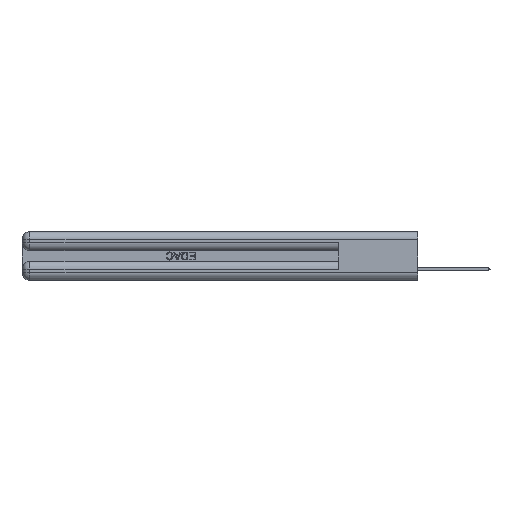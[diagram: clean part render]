
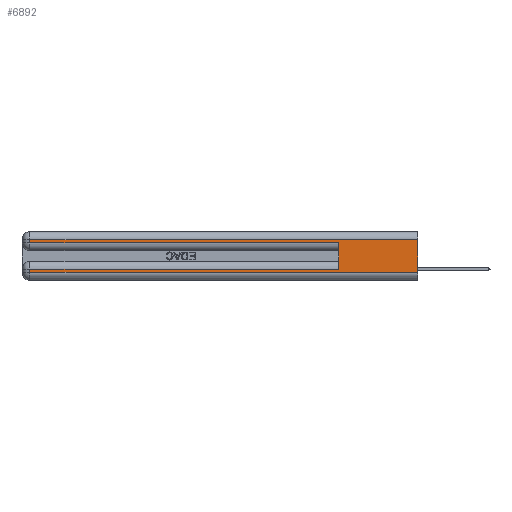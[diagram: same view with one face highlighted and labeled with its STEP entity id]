
A CAD part, left-side view. The second image highlights one B-rep face of the part: STEP entity #6892.
In plain terms, the highlighted planar face has unit normal (-1, 0, 0).
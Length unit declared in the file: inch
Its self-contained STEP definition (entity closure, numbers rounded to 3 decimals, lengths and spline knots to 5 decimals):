
#1391 = DIRECTION ( 'NONE',  ( 0., 0., -1. ) ) ;
#2297 = CARTESIAN_POINT ( 'NONE',  ( 0., 0., 0.37 ) ) ;
#4176 = VECTOR ( 'NONE', #13015, 39.37008 ) ;
#6459 = EDGE_CURVE ( 'NONE', #27308, #42608, #42699, .T. ) ;
#6892 = ADVANCED_FACE ( 'NONE', ( #25023 ), #39674, .F. ) ;
#7155 = CARTESIAN_POINT ( 'NONE',  ( 0., 0., 0.31 ) ) ;
#7346 = CARTESIAN_POINT ( 'NONE',  ( 0., 0.6, 0.285 ) ) ;
#7790 = ORIENTED_EDGE ( 'NONE', *, *, #52437, .F. ) ;
#8137 = EDGE_LOOP ( 'NONE', ( #46172, #17367, #47020, #34100, #7790, #23976, #26842, #10623 ) ) ;
#8262 = VECTOR ( 'NONE', #26020, 39.37008 ) ;
#9914 = CARTESIAN_POINT ( 'NONE',  ( 0., 0., 0.37 ) ) ;
#9934 = CARTESIAN_POINT ( 'NONE',  ( 0., 2.94, 0.285 ) ) ;
#10623 = ORIENTED_EDGE ( 'NONE', *, *, #6459, .T. ) ;
#12731 = EDGE_CURVE ( 'NONE', #39563, #20555, #53497, .T. ) ;
#12941 = CARTESIAN_POINT ( 'NONE',  ( 0., 0., 0.085 ) ) ;
#13015 = DIRECTION ( 'NONE',  ( 0., -1., 0. ) ) ;
#13288 = LINE ( 'NONE', #42348, #19862 ) ;
#13444 = LINE ( 'NONE', #12941, #14141 ) ;
#14141 = VECTOR ( 'NONE', #50547, 39.37008 ) ;
#14188 = VECTOR ( 'NONE', #1391, 39.37008 ) ;
#14532 = DIRECTION ( 'NONE',  ( 1., 0., 0. ) ) ;
#17285 = CARTESIAN_POINT ( 'NONE',  ( 0., 0.6, 0.145 ) ) ;
#17367 = ORIENTED_EDGE ( 'NONE', *, *, #12731, .T. ) ;
#17448 = EDGE_CURVE ( 'NONE', #20555, #49701, #46870, .T. ) ;
#17715 = CARTESIAN_POINT ( 'NONE',  ( 0., 0.6, 0.085 ) ) ;
#18235 = CARTESIAN_POINT ( 'NONE',  ( 0., 0., 0.285 ) ) ;
#18261 = EDGE_CURVE ( 'NONE', #46869, #44835, #13444, .T. ) ;
#18757 = LINE ( 'NONE', #17285, #8262 ) ;
#18888 = DIRECTION ( 'NONE',  ( 0., 0., -1. ) ) ;
#19402 = CARTESIAN_POINT ( 'NONE',  ( 0., 2.94, 0.31 ) ) ;
#19862 = VECTOR ( 'NONE', #25719, 39.37008 ) ;
#20555 = VERTEX_POINT ( 'NONE', #19402 ) ;
#23053 = AXIS2_PLACEMENT_3D ( 'NONE', #2297, #14532, #18888 ) ;
#23287 = LINE ( 'NONE', #9914, #24608 ) ;
#23378 = DIRECTION ( 'NONE',  ( 0., -1., 0. ) ) ;
#23976 = ORIENTED_EDGE ( 'NONE', *, *, #18261, .T. ) ;
#24017 = CARTESIAN_POINT ( 'NONE',  ( 0., 0., 0.31 ) ) ;
#24608 = VECTOR ( 'NONE', #39109, 39.37008 ) ;
#25023 = FACE_OUTER_BOUND ( 'NONE', #8137, .T. ) ;
#25719 = DIRECTION ( 'NONE',  ( 0., 0., -1. ) ) ;
#26020 = DIRECTION ( 'NONE',  ( 0., 0., 1. ) ) ;
#26842 = ORIENTED_EDGE ( 'NONE', *, *, #28242, .T. ) ;
#27308 = VERTEX_POINT ( 'NONE', #29574 ) ;
#28242 = EDGE_CURVE ( 'NONE', #44835, #27308, #13288, .T. ) ;
#28376 = LINE ( 'NONE', #18235, #38136 ) ;
#28681 = DIRECTION ( 'NONE',  ( 0., 1., 0. ) ) ;
#29574 = CARTESIAN_POINT ( 'NONE',  ( 0., 2.94, 0.06 ) ) ;
#31251 = VECTOR ( 'NONE', #28681, 39.37008 ) ;
#34100 = ORIENTED_EDGE ( 'NONE', *, *, #40107, .T. ) ;
#36071 = CARTESIAN_POINT ( 'NONE',  ( 0., 2.94, 0.085 ) ) ;
#37442 = EDGE_CURVE ( 'NONE', #39563, #42608, #23287, .T. ) ;
#38136 = VECTOR ( 'NONE', #23378, 39.37008 ) ;
#39109 = DIRECTION ( 'NONE',  ( 0., 0., -1. ) ) ;
#39563 = VERTEX_POINT ( 'NONE', #24017 ) ;
#39674 = PLANE ( 'NONE',  #23053 ) ;
#40107 = EDGE_CURVE ( 'NONE', #49701, #51610, #28376, .T. ) ;
#42348 = CARTESIAN_POINT ( 'NONE',  ( 0., 2.94, 0.37 ) ) ;
#42608 = VERTEX_POINT ( 'NONE', #47594 ) ;
#42699 = LINE ( 'NONE', #43984, #4176 ) ;
#43984 = CARTESIAN_POINT ( 'NONE',  ( 0., 0., 0.06 ) ) ;
#44835 = VERTEX_POINT ( 'NONE', #36071 ) ;
#46172 = ORIENTED_EDGE ( 'NONE', *, *, #37442, .F. ) ;
#46869 = VERTEX_POINT ( 'NONE', #17715 ) ;
#46870 = LINE ( 'NONE', #51199, #14188 ) ;
#47020 = ORIENTED_EDGE ( 'NONE', *, *, #17448, .T. ) ;
#47594 = CARTESIAN_POINT ( 'NONE',  ( 0., 0., 0.06 ) ) ;
#49701 = VERTEX_POINT ( 'NONE', #9934 ) ;
#50547 = DIRECTION ( 'NONE',  ( 0., 1., 0. ) ) ;
#51199 = CARTESIAN_POINT ( 'NONE',  ( 0., 2.94, 0.37 ) ) ;
#51610 = VERTEX_POINT ( 'NONE', #7346 ) ;
#52437 = EDGE_CURVE ( 'NONE', #46869, #51610, #18757, .T. ) ;
#53497 = LINE ( 'NONE', #7155, #31251 ) ;
